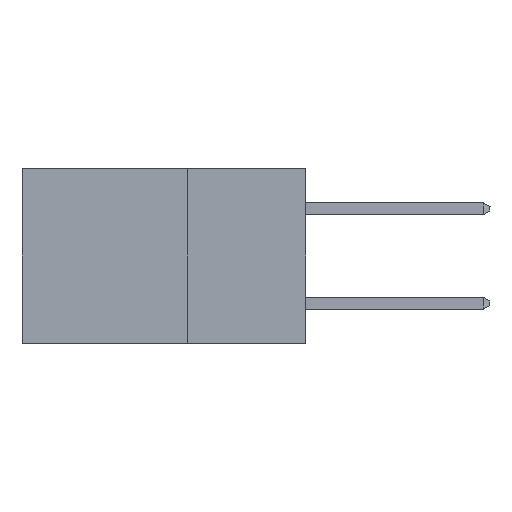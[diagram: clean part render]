
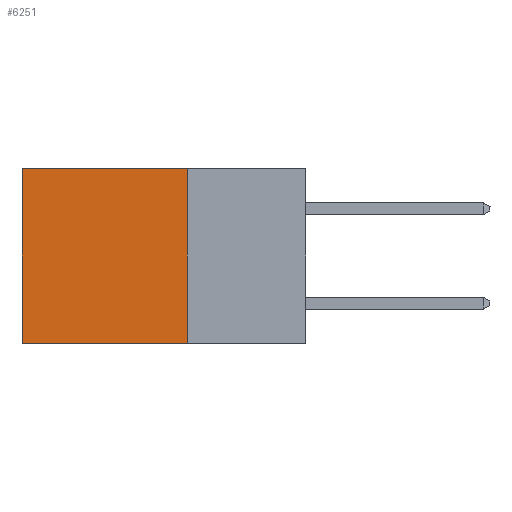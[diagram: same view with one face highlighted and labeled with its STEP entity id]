
A CAD part, left-side view. The second image highlights one B-rep face of the part: STEP entity #6251.
In plain terms, the highlighted planar face has unit normal (-1, 0, 0).
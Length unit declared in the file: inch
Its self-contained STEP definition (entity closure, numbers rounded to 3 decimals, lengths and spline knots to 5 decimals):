
#79 = CARTESIAN_POINT ( 'NONE',  ( 0.298, 0.6, -0.37 ) ) ;
#102 = ORIENTED_EDGE ( 'NONE', *, *, #12039, .T. ) ;
#195 = VECTOR ( 'NONE', #7872, 39.37008 ) ;
#608 = VERTEX_POINT ( 'NONE', #11845 ) ;
#936 = DIRECTION ( 'NONE',  ( 0., 0., -1. ) ) ;
#1941 = ORIENTED_EDGE ( 'NONE', *, *, #17298, .T. ) ;
#2465 = FACE_OUTER_BOUND ( 'NONE', #21756, .T. ) ;
#2468 = DIRECTION ( 'NONE',  ( 0., 1., 0. ) ) ;
#3242 = CARTESIAN_POINT ( 'NONE',  ( 0.298, 0.25, 0. ) ) ;
#3558 = ORIENTED_EDGE ( 'NONE', *, *, #7988, .F. ) ;
#5231 = DIRECTION ( 'NONE',  ( 1., 0., 0. ) ) ;
#5721 = ORIENTED_EDGE ( 'NONE', *, *, #18580, .F. ) ;
#5722 = VECTOR ( 'NONE', #2468, 39.37008 ) ;
#6251 = ADVANCED_FACE ( 'NONE', ( #2465 ), #25817, .F. ) ;
#6903 = LINE ( 'NONE', #8899, #11613 ) ;
#7872 = DIRECTION ( 'NONE',  ( 0., 1., 0. ) ) ;
#7988 = EDGE_CURVE ( 'NONE', #608, #25912, #14239, .T. ) ;
#8899 = CARTESIAN_POINT ( 'NONE',  ( 0.298, 0.6, 0. ) ) ;
#9872 = VECTOR ( 'NONE', #12991, 39.37008 ) ;
#11613 = VECTOR ( 'NONE', #936, 39.37008 ) ;
#11845 = CARTESIAN_POINT ( 'NONE',  ( 0.298, 0.25, 0. ) ) ;
#12039 = EDGE_CURVE ( 'NONE', #608, #21538, #20280, .T. ) ;
#12991 = DIRECTION ( 'NONE',  ( 0., 0., -1. ) ) ;
#13212 = CARTESIAN_POINT ( 'NONE',  ( 0.298, 0.6, 0. ) ) ;
#14239 = LINE ( 'NONE', #25065, #9872 ) ;
#15069 = DIRECTION ( 'NONE',  ( 0., 0., -1. ) ) ;
#15358 = CARTESIAN_POINT ( 'NONE',  ( 0.298, 0.25, -0.37 ) ) ;
#16140 = AXIS2_PLACEMENT_3D ( 'NONE', #3242, #5231, #15069 ) ;
#17298 = EDGE_CURVE ( 'NONE', #21538, #21078, #6903, .T. ) ;
#17356 = LINE ( 'NONE', #22221, #5722 ) ;
#18580 = EDGE_CURVE ( 'NONE', #25912, #21078, #17356, .T. ) ;
#20280 = LINE ( 'NONE', #24067, #195 ) ;
#21078 = VERTEX_POINT ( 'NONE', #79 ) ;
#21538 = VERTEX_POINT ( 'NONE', #13212 ) ;
#21756 = EDGE_LOOP ( 'NONE', ( #1941, #5721, #3558, #102 ) ) ;
#22221 = CARTESIAN_POINT ( 'NONE',  ( 0.298, 0.25, -0.37 ) ) ;
#24067 = CARTESIAN_POINT ( 'NONE',  ( 0.298, 0.25, 0. ) ) ;
#25065 = CARTESIAN_POINT ( 'NONE',  ( 0.298, 0.25, 0. ) ) ;
#25817 = PLANE ( 'NONE',  #16140 ) ;
#25912 = VERTEX_POINT ( 'NONE', #15358 ) ;
